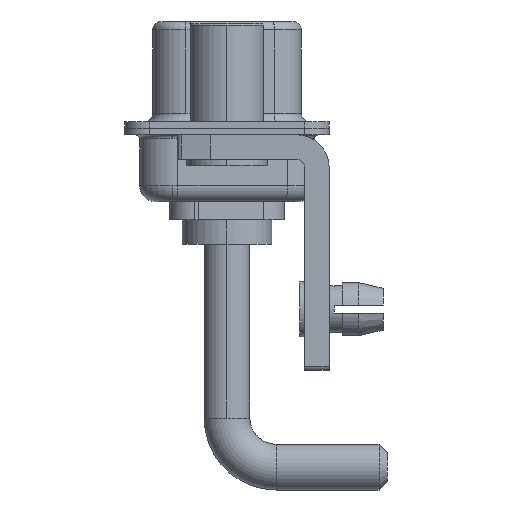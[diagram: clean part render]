
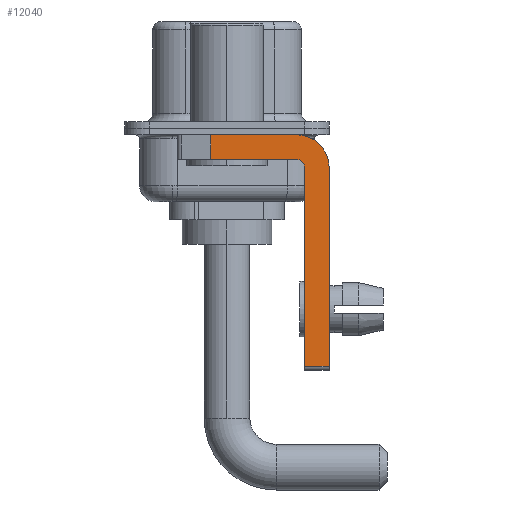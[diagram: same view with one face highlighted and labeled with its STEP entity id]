
A CAD part, left-side view. The second image highlights one B-rep face of the part: STEP entity #12040.
In plain terms, the highlighted planar face has unit normal (-1, 0, 0).
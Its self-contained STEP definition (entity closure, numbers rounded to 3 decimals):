
#123 = CARTESIAN_POINT ( 'NONE',  ( -2.9, 0.978, -0.4 ) ) ;
#344 = DIRECTION ( 'NONE',  ( 1., 0., 0. ) ) ;
#628 = CARTESIAN_POINT ( 'NONE',  ( -2.9, -4.25, -1.9 ) ) ;
#780 = EDGE_LOOP ( 'NONE', ( #1427, #4791, #10781, #2880, #5719, #8617, #15360, #2600 ) ) ;
#804 = DIRECTION ( 'NONE',  ( 0., 0., -1. ) ) ;
#955 = CARTESIAN_POINT ( 'NONE',  ( -2.9, 0.978, -1.9 ) ) ;
#1231 = CARTESIAN_POINT ( 'NONE',  ( -2.9, -4.25, -0.4 ) ) ;
#1291 = AXIS2_PLACEMENT_3D ( 'NONE', #5643, #344, #13204 ) ;
#1348 = CARTESIAN_POINT ( 'NONE',  ( -2.9, -6.25, -14.55 ) ) ;
#1427 = ORIENTED_EDGE ( 'NONE', *, *, #5148, .F. ) ;
#2071 = AXIS2_PLACEMENT_3D ( 'NONE', #16716, #3103, #15177 ) ;
#2558 = EDGE_CURVE ( 'NONE', #10191, #8700, #19771, .T. ) ;
#2600 = ORIENTED_EDGE ( 'NONE', *, *, #17151, .F. ) ;
#2715 = VECTOR ( 'NONE', #14493, 1000. ) ;
#2880 = ORIENTED_EDGE ( 'NONE', *, *, #8369, .F. ) ;
#3103 = DIRECTION ( 'NONE',  ( 1., 0., 0. ) ) ;
#3604 = DIRECTION ( 'NONE',  ( 0., 1., 0. ) ) ;
#3872 = PLANE ( 'NONE',  #1291 ) ;
#4421 = VERTEX_POINT ( 'NONE', #1231 ) ;
#4791 = ORIENTED_EDGE ( 'NONE', *, *, #10529, .T. ) ;
#5148 = EDGE_CURVE ( 'NONE', #6222, #4421, #8253, .T. ) ;
#5643 = CARTESIAN_POINT ( 'NONE',  ( -2.9, -4.25, -2.4 ) ) ;
#5719 = ORIENTED_EDGE ( 'NONE', *, *, #2558, .F. ) ;
#5952 = LINE ( 'NONE', #7264, #9620 ) ;
#5999 = VERTEX_POINT ( 'NONE', #955 ) ;
#6154 = CIRCLE ( 'NONE', #15933, 0.5 ) ;
#6222 = VERTEX_POINT ( 'NONE', #123 ) ;
#6474 = VERTEX_POINT ( 'NONE', #628 ) ;
#7264 = CARTESIAN_POINT ( 'NONE',  ( -2.9, -4.25, -14.55 ) ) ;
#7699 = DIRECTION ( 'NONE',  ( 0., 0., 1. ) ) ;
#8253 = LINE ( 'NONE', #12882, #2715 ) ;
#8369 = EDGE_CURVE ( 'NONE', #8700, #6474, #6154, .T. ) ;
#8599 = CIRCLE ( 'NONE', #2071, 2. ) ;
#8617 = ORIENTED_EDGE ( 'NONE', *, *, #17523, .T. ) ;
#8700 = VERTEX_POINT ( 'NONE', #17717 ) ;
#8750 = EDGE_CURVE ( 'NONE', #6474, #5999, #11302, .T. ) ;
#8801 = FACE_OUTER_BOUND ( 'NONE', #780, .T. ) ;
#8833 = CARTESIAN_POINT ( 'NONE',  ( -2.9, -4.75, -14.8 ) ) ;
#9536 = EDGE_CURVE ( 'NONE', #12523, #15900, #11764, .T. ) ;
#9620 = VECTOR ( 'NONE', #18407, 1000. ) ;
#10144 = CARTESIAN_POINT ( 'NONE',  ( -2.9, -4.25, -1.9 ) ) ;
#10191 = VERTEX_POINT ( 'NONE', #17242 ) ;
#10529 = EDGE_CURVE ( 'NONE', #6222, #5999, #14718, .T. ) ;
#10613 = CARTESIAN_POINT ( 'NONE',  ( -2.9, -6.25, -2.4 ) ) ;
#10781 = ORIENTED_EDGE ( 'NONE', *, *, #8750, .F. ) ;
#11302 = LINE ( 'NONE', #10144, #11721 ) ;
#11474 = DIRECTION ( 'NONE',  ( 0., 0., -1. ) ) ;
#11721 = VECTOR ( 'NONE', #3604, 1000. ) ;
#11764 = LINE ( 'NONE', #14811, #15932 ) ;
#12040 = ADVANCED_FACE ( 'NONE', ( #8801 ), #3872, .F. ) ;
#12523 = VERTEX_POINT ( 'NONE', #10613 ) ;
#12882 = CARTESIAN_POINT ( 'NONE',  ( -2.9, 3., -0.4 ) ) ;
#13198 = CARTESIAN_POINT ( 'NONE',  ( -2.9, 0.978, -1.9 ) ) ;
#13204 = DIRECTION ( 'NONE',  ( 0., 0., -1. ) ) ;
#14453 = VECTOR ( 'NONE', #15049, 1000. ) ;
#14493 = DIRECTION ( 'NONE',  ( 0., -1., 0. ) ) ;
#14718 = LINE ( 'NONE', #13198, #19901 ) ;
#14811 = CARTESIAN_POINT ( 'NONE',  ( -2.9, -6.25, -2.4 ) ) ;
#15049 = DIRECTION ( 'NONE',  ( 0., 0., 1. ) ) ;
#15177 = DIRECTION ( 'NONE',  ( 0., 0., -1. ) ) ;
#15360 = ORIENTED_EDGE ( 'NONE', *, *, #9536, .F. ) ;
#15666 = DIRECTION ( 'NONE',  ( -1., 0., 0. ) ) ;
#15900 = VERTEX_POINT ( 'NONE', #1348 ) ;
#15932 = VECTOR ( 'NONE', #804, 1000. ) ;
#15933 = AXIS2_PLACEMENT_3D ( 'NONE', #18750, #15666, #7699 ) ;
#16716 = CARTESIAN_POINT ( 'NONE',  ( -2.9, -4.25, -2.4 ) ) ;
#17151 = EDGE_CURVE ( 'NONE', #4421, #12523, #8599, .T. ) ;
#17242 = CARTESIAN_POINT ( 'NONE',  ( -2.9, -4.75, -14.55 ) ) ;
#17523 = EDGE_CURVE ( 'NONE', #10191, #15900, #5952, .T. ) ;
#17717 = CARTESIAN_POINT ( 'NONE',  ( -2.9, -4.75, -2.4 ) ) ;
#18407 = DIRECTION ( 'NONE',  ( 0., -1., 0. ) ) ;
#18750 = CARTESIAN_POINT ( 'NONE',  ( -2.9, -4.25, -2.4 ) ) ;
#19771 = LINE ( 'NONE', #8833, #14453 ) ;
#19901 = VECTOR ( 'NONE', #11474, 1000. ) ;
